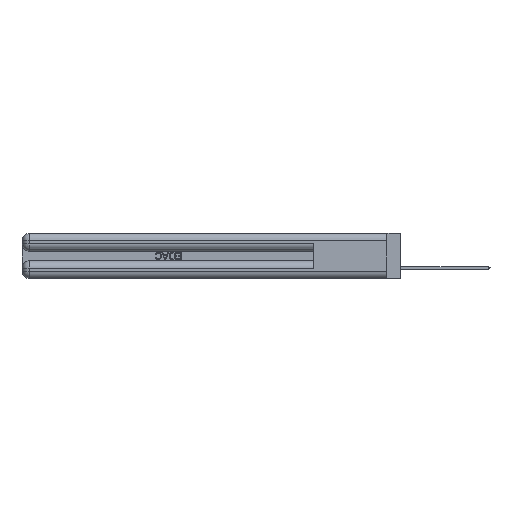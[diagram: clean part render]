
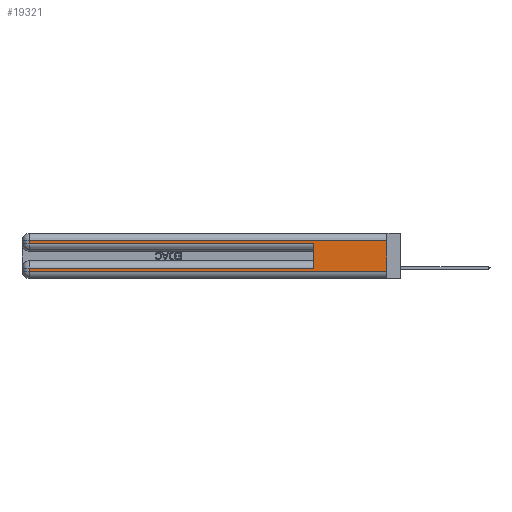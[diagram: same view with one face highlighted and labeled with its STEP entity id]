
A CAD part, left-side view. The second image highlights one B-rep face of the part: STEP entity #19321.
In plain terms, the highlighted planar face has unit normal (-1, 0, 0).
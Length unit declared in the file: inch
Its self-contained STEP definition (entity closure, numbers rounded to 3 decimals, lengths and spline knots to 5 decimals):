
#2182 = VERTEX_POINT ( 'NONE', #16545 ) ;
#3709 = CARTESIAN_POINT ( 'NONE',  ( 0., 0., 0.285 ) ) ;
#3889 = ORIENTED_EDGE ( 'NONE', *, *, #21484, .T. ) ;
#4473 = ORIENTED_EDGE ( 'NONE', *, *, #50396, .T. ) ;
#4780 = EDGE_CURVE ( 'NONE', #52742, #35582, #8216, .T. ) ;
#6293 = VECTOR ( 'NONE', #15991, 39.37008 ) ;
#6442 = ORIENTED_EDGE ( 'NONE', *, *, #42550, .F. ) ;
#7655 = CARTESIAN_POINT ( 'NONE',  ( 0., 0., 0.37 ) ) ;
#7884 = LINE ( 'NONE', #32786, #40360 ) ;
#8073 = EDGE_CURVE ( 'NONE', #2182, #35582, #43046, .T. ) ;
#8212 = VERTEX_POINT ( 'NONE', #31338 ) ;
#8216 = LINE ( 'NONE', #3709, #6293 ) ;
#9100 = VECTOR ( 'NONE', #44373, 39.37008 ) ;
#9363 = VECTOR ( 'NONE', #11602, 39.37008 ) ;
#11602 = DIRECTION ( 'NONE',  ( 0., 1., 0. ) ) ;
#12261 = AXIS2_PLACEMENT_3D ( 'NONE', #7655, #32213, #48379 ) ;
#12408 = PLANE ( 'NONE',  #12261 ) ;
#15816 = EDGE_LOOP ( 'NONE', ( #6442, #3889, #24583, #42128, #38569, #52256, #4473, #41108 ) ) ;
#15991 = DIRECTION ( 'NONE',  ( 0., -1., 0. ) ) ;
#16545 = CARTESIAN_POINT ( 'NONE',  ( 0., 0.6, 0.085 ) ) ;
#17127 = CARTESIAN_POINT ( 'NONE',  ( 0., 0.6, 0.285 ) ) ;
#18016 = EDGE_CURVE ( 'NONE', #8212, #36453, #45421, .T. ) ;
#19321 = ADVANCED_FACE ( 'NONE', ( #51034 ), #12408, .F. ) ;
#19578 = CARTESIAN_POINT ( 'NONE',  ( 0., 0.6, 0.145 ) ) ;
#21484 = EDGE_CURVE ( 'NONE', #47408, #38702, #41238, .T. ) ;
#23794 = CARTESIAN_POINT ( 'NONE',  ( 0., 2.94, 0.31 ) ) ;
#24022 = VERTEX_POINT ( 'NONE', #30431 ) ;
#24167 = CARTESIAN_POINT ( 'NONE',  ( 0., 0., 0.085 ) ) ;
#24583 = ORIENTED_EDGE ( 'NONE', *, *, #47981, .T. ) ;
#25559 = LINE ( 'NONE', #27292, #38977 ) ;
#27292 = CARTESIAN_POINT ( 'NONE',  ( 0., 2.94, 0.37 ) ) ;
#28107 = DIRECTION ( 'NONE',  ( 0., 0., -1. ) ) ;
#28189 = DIRECTION ( 'NONE',  ( 0., 1., 0. ) ) ;
#30431 = CARTESIAN_POINT ( 'NONE',  ( 0., 2.94, 0.085 ) ) ;
#31338 = CARTESIAN_POINT ( 'NONE',  ( 0., 2.94, 0.06 ) ) ;
#32213 = DIRECTION ( 'NONE',  ( 1., 0., 0. ) ) ;
#32639 = DIRECTION ( 'NONE',  ( 0., 0., -1. ) ) ;
#32786 = CARTESIAN_POINT ( 'NONE',  ( 0., 0., 0.37 ) ) ;
#33148 = VECTOR ( 'NONE', #28189, 39.37008 ) ;
#33444 = CARTESIAN_POINT ( 'NONE',  ( 0., 2.94, 0.285 ) ) ;
#34305 = CARTESIAN_POINT ( 'NONE',  ( 0., 0., 0.06 ) ) ;
#35582 = VERTEX_POINT ( 'NONE', #17127 ) ;
#36453 = VERTEX_POINT ( 'NONE', #34305 ) ;
#37614 = DIRECTION ( 'NONE',  ( 0., 0., 1. ) ) ;
#38569 = ORIENTED_EDGE ( 'NONE', *, *, #8073, .F. ) ;
#38702 = VERTEX_POINT ( 'NONE', #23794 ) ;
#38807 = DIRECTION ( 'NONE',  ( 0., 0., -1. ) ) ;
#38977 = VECTOR ( 'NONE', #38807, 39.37008 ) ;
#39438 = CARTESIAN_POINT ( 'NONE',  ( 0., 0., 0.31 ) ) ;
#39734 = CARTESIAN_POINT ( 'NONE',  ( 0., 0., 0.06 ) ) ;
#39876 = CARTESIAN_POINT ( 'NONE',  ( 0., 0., 0.31 ) ) ;
#40360 = VECTOR ( 'NONE', #32639, 39.37008 ) ;
#41108 = ORIENTED_EDGE ( 'NONE', *, *, #18016, .T. ) ;
#41238 = LINE ( 'NONE', #39876, #9363 ) ;
#42128 = ORIENTED_EDGE ( 'NONE', *, *, #4780, .T. ) ;
#42550 = EDGE_CURVE ( 'NONE', #47408, #36453, #7884, .T. ) ;
#43046 = LINE ( 'NONE', #19578, #51335 ) ;
#44100 = CARTESIAN_POINT ( 'NONE',  ( 0., 2.94, 0.37 ) ) ;
#44373 = DIRECTION ( 'NONE',  ( 0., -1., 0. ) ) ;
#45421 = LINE ( 'NONE', #39734, #9100 ) ;
#45815 = LINE ( 'NONE', #24167, #33148 ) ;
#47408 = VERTEX_POINT ( 'NONE', #39438 ) ;
#47981 = EDGE_CURVE ( 'NONE', #38702, #52742, #25559, .T. ) ;
#48379 = DIRECTION ( 'NONE',  ( 0., 0., -1. ) ) ;
#48606 = VECTOR ( 'NONE', #28107, 39.37008 ) ;
#50396 = EDGE_CURVE ( 'NONE', #24022, #8212, #51143, .T. ) ;
#51034 = FACE_OUTER_BOUND ( 'NONE', #15816, .T. ) ;
#51143 = LINE ( 'NONE', #44100, #48606 ) ;
#51335 = VECTOR ( 'NONE', #37614, 39.37008 ) ;
#51751 = EDGE_CURVE ( 'NONE', #2182, #24022, #45815, .T. ) ;
#52256 = ORIENTED_EDGE ( 'NONE', *, *, #51751, .T. ) ;
#52742 = VERTEX_POINT ( 'NONE', #33444 ) ;
